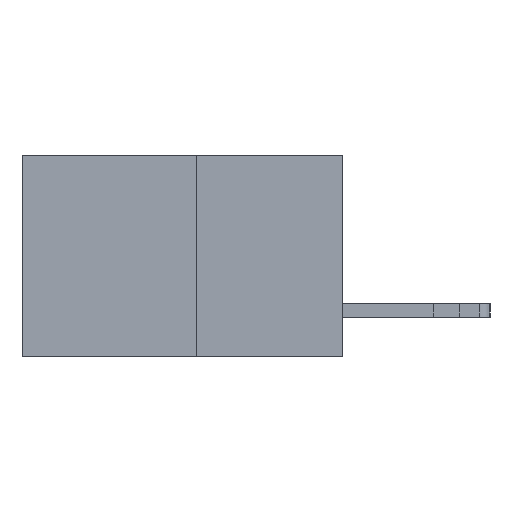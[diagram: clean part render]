
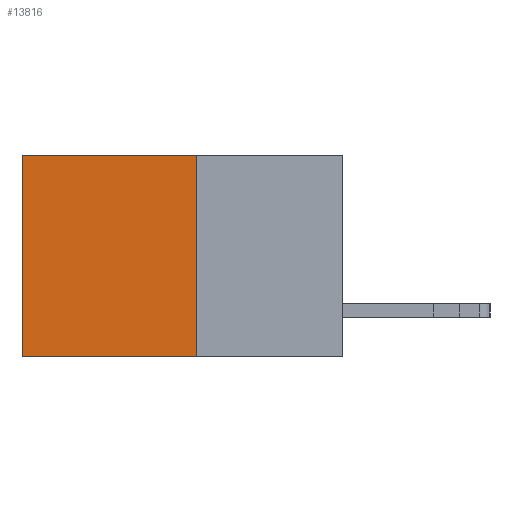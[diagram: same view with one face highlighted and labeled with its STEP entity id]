
A CAD part, left-side view. The second image highlights one B-rep face of the part: STEP entity #13816.
In plain terms, the highlighted planar face has unit normal (-1, 0, 0).
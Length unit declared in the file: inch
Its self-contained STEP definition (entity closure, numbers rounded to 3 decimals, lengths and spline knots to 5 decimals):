
#152 = ORIENTED_EDGE ( 'NONE', *, *, #7317, .T. ) ;
#268 = LINE ( 'NONE', #15470, #11353 ) ;
#771 = CARTESIAN_POINT ( 'NONE',  ( 0.277, 0.27, -0.37 ) ) ;
#1536 = DIRECTION ( 'NONE',  ( 0., 1., 0. ) ) ;
#1769 = CARTESIAN_POINT ( 'NONE',  ( 0.277, 0.59, -0.37 ) ) ;
#1842 = DIRECTION ( 'NONE',  ( 1., 0., 0. ) ) ;
#2815 = VERTEX_POINT ( 'NONE', #3276 ) ;
#3276 = CARTESIAN_POINT ( 'NONE',  ( 0.277, 0.27, -0.37 ) ) ;
#3957 = LINE ( 'NONE', #8763, #17869 ) ;
#4054 = EDGE_CURVE ( 'NONE', #2815, #4929, #268, .T. ) ;
#4239 = LINE ( 'NONE', #11287, #11274 ) ;
#4929 = VERTEX_POINT ( 'NONE', #1769 ) ;
#5317 = ORIENTED_EDGE ( 'NONE', *, *, #9363, .T. ) ;
#5605 = LINE ( 'NONE', #771, #9773 ) ;
#5780 = EDGE_CURVE ( 'NONE', #6068, #2815, #5605, .T. ) ;
#6068 = VERTEX_POINT ( 'NONE', #12776 ) ;
#6226 = DIRECTION ( 'NONE',  ( 0., 1., 0. ) ) ;
#6725 = ORIENTED_EDGE ( 'NONE', *, *, #4054, .F. ) ;
#7317 = EDGE_CURVE ( 'NONE', #6068, #10106, #3957, .T. ) ;
#8563 = DIRECTION ( 'NONE',  ( 0., 0., -1. ) ) ;
#8763 = CARTESIAN_POINT ( 'NONE',  ( 0.277, 0.27, 0. ) ) ;
#9239 = AXIS2_PLACEMENT_3D ( 'NONE', #15696, #1842, #11792 ) ;
#9363 = EDGE_CURVE ( 'NONE', #10106, #4929, #4239, .T. ) ;
#9773 = VECTOR ( 'NONE', #16073, 39.37008 ) ;
#10106 = VERTEX_POINT ( 'NONE', #17838 ) ;
#10471 = PLANE ( 'NONE',  #9239 ) ;
#11274 = VECTOR ( 'NONE', #8563, 39.37008 ) ;
#11287 = CARTESIAN_POINT ( 'NONE',  ( 0.277, 0.59, -0.37 ) ) ;
#11353 = VECTOR ( 'NONE', #6226, 39.37008 ) ;
#11792 = DIRECTION ( 'NONE',  ( 0., 0., -1. ) ) ;
#12372 = FACE_OUTER_BOUND ( 'NONE', #12922, .T. ) ;
#12776 = CARTESIAN_POINT ( 'NONE',  ( 0.277, 0.27, 0. ) ) ;
#12922 = EDGE_LOOP ( 'NONE', ( #5317, #6725, #14686, #152 ) ) ;
#13816 = ADVANCED_FACE ( 'NONE', ( #12372 ), #10471, .F. ) ;
#14686 = ORIENTED_EDGE ( 'NONE', *, *, #5780, .F. ) ;
#15470 = CARTESIAN_POINT ( 'NONE',  ( 0.277, 0.27, -0.37 ) ) ;
#15696 = CARTESIAN_POINT ( 'NONE',  ( 0.277, 0.27, -0.37 ) ) ;
#16073 = DIRECTION ( 'NONE',  ( 0., 0., -1. ) ) ;
#17838 = CARTESIAN_POINT ( 'NONE',  ( 0.277, 0.59, 0. ) ) ;
#17869 = VECTOR ( 'NONE', #1536, 39.37008 ) ;
